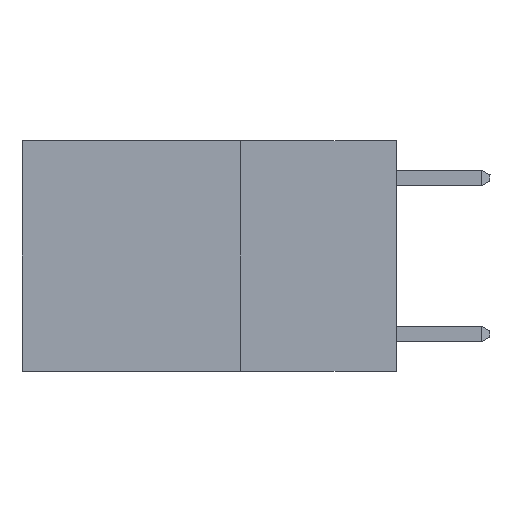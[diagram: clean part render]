
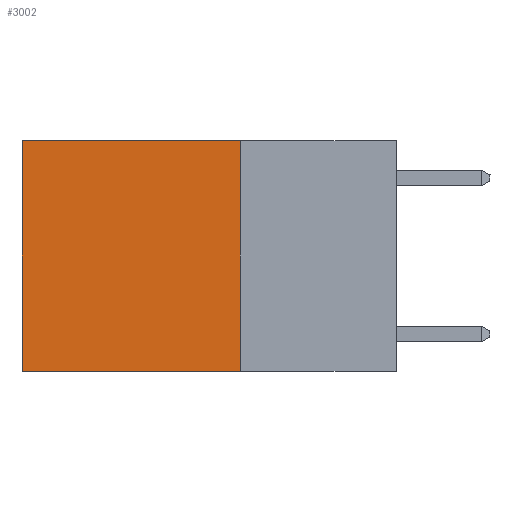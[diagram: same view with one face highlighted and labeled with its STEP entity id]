
A CAD part, left-side view. The second image highlights one B-rep face of the part: STEP entity #3002.
In plain terms, the highlighted planar face has unit normal (-1, 0, 0).
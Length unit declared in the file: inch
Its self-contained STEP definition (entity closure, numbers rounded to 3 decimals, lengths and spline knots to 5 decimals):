
#58 = CARTESIAN_POINT ( 'NONE',  ( 0.2625, 0.25, 0. ) ) ;
#1117 = CARTESIAN_POINT ( 'NONE',  ( 0.2625, 0.6, 0. ) ) ;
#1344 = DIRECTION ( 'NONE',  ( 0., 0., -1. ) ) ;
#2412 = LINE ( 'NONE', #10928, #10641 ) ;
#2566 = VECTOR ( 'NONE', #12361, 39.37008 ) ;
#3002 = ADVANCED_FACE ( 'NONE', ( #6082 ), #12082, .F. ) ;
#3079 = VERTEX_POINT ( 'NONE', #6234 ) ;
#3301 = ORIENTED_EDGE ( 'NONE', *, *, #10498, .F. ) ;
#3438 = VERTEX_POINT ( 'NONE', #4825 ) ;
#3666 = LINE ( 'NONE', #1117, #10710 ) ;
#4825 = CARTESIAN_POINT ( 'NONE',  ( 0.2625, 0.25, 0. ) ) ;
#5487 = VERTEX_POINT ( 'NONE', #6900 ) ;
#5879 = ORIENTED_EDGE ( 'NONE', *, *, #8617, .T. ) ;
#6082 = FACE_OUTER_BOUND ( 'NONE', #6526, .T. ) ;
#6234 = CARTESIAN_POINT ( 'NONE',  ( 0.2625, 0.6, -0.37 ) ) ;
#6504 = EDGE_CURVE ( 'NONE', #5487, #3079, #3666, .T. ) ;
#6526 = EDGE_LOOP ( 'NONE', ( #13589, #6955, #3301, #5879 ) ) ;
#6900 = CARTESIAN_POINT ( 'NONE',  ( 0.2625, 0.6, 0. ) ) ;
#6955 = ORIENTED_EDGE ( 'NONE', *, *, #9233, .F. ) ;
#7622 = CARTESIAN_POINT ( 'NONE',  ( 0.2625, 0.25, 0. ) ) ;
#8289 = DIRECTION ( 'NONE',  ( 0., 0., -1. ) ) ;
#8617 = EDGE_CURVE ( 'NONE', #3438, #5487, #14542, .T. ) ;
#8676 = DIRECTION ( 'NONE',  ( 0., 0., -1. ) ) ;
#8994 = VECTOR ( 'NONE', #8289, 39.37008 ) ;
#9233 = EDGE_CURVE ( 'NONE', #10352, #3079, #2412, .T. ) ;
#10352 = VERTEX_POINT ( 'NONE', #13733 ) ;
#10498 = EDGE_CURVE ( 'NONE', #3438, #10352, #11878, .T. ) ;
#10641 = VECTOR ( 'NONE', #12009, 39.37008 ) ;
#10710 = VECTOR ( 'NONE', #1344, 39.37008 ) ;
#10928 = CARTESIAN_POINT ( 'NONE',  ( 0.2625, 0.25, -0.37 ) ) ;
#11878 = LINE ( 'NONE', #58, #8994 ) ;
#12009 = DIRECTION ( 'NONE',  ( 0., 1., 0. ) ) ;
#12082 = PLANE ( 'NONE',  #15339 ) ;
#12229 = DIRECTION ( 'NONE',  ( 1., 0., 0. ) ) ;
#12361 = DIRECTION ( 'NONE',  ( 0., 1., 0. ) ) ;
#13210 = CARTESIAN_POINT ( 'NONE',  ( 0.2625, 0.25, 0. ) ) ;
#13589 = ORIENTED_EDGE ( 'NONE', *, *, #6504, .T. ) ;
#13733 = CARTESIAN_POINT ( 'NONE',  ( 0.2625, 0.25, -0.37 ) ) ;
#14542 = LINE ( 'NONE', #7622, #2566 ) ;
#15339 = AXIS2_PLACEMENT_3D ( 'NONE', #13210, #12229, #8676 ) ;
